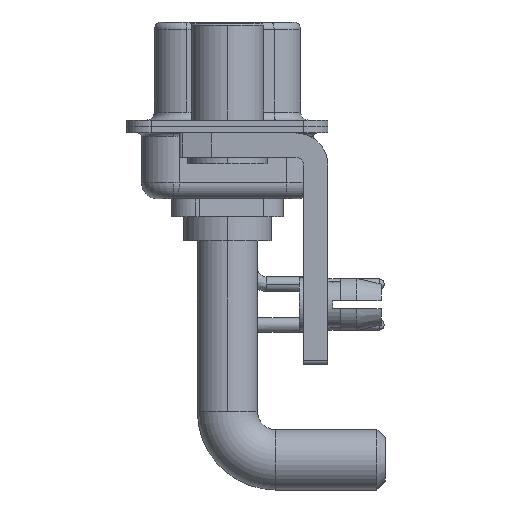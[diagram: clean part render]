
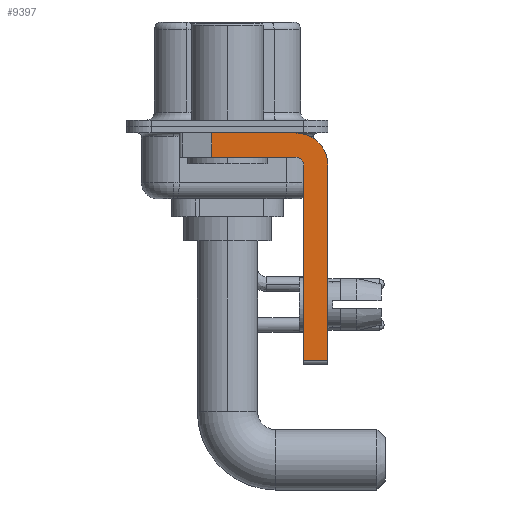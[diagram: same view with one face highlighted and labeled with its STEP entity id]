
A CAD part, left-side view. The second image highlights one B-rep face of the part: STEP entity #9397.
In plain terms, the highlighted planar face has unit normal (-1, 0, 0).
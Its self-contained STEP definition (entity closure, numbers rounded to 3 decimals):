
#890 = EDGE_CURVE ( 'NONE', #4836, #10333, #4775, .T. ) ;
#1061 = LINE ( 'NONE', #7834, #28828 ) ;
#1086 = VECTOR ( 'NONE', #16494, 1000. ) ;
#1589 = VECTOR ( 'NONE', #26887, 1000. ) ;
#1786 = CARTESIAN_POINT ( 'NONE',  ( -2.9, -6.25, -2.4 ) ) ;
#2987 = VECTOR ( 'NONE', #22084, 1000. ) ;
#4348 = CARTESIAN_POINT ( 'NONE',  ( -2.9, 0.978, -0.4 ) ) ;
#4496 = EDGE_CURVE ( 'NONE', #12629, #29725, #12776, .T. ) ;
#4773 = VERTEX_POINT ( 'NONE', #27335 ) ;
#4775 = LINE ( 'NONE', #1786, #22903 ) ;
#4836 = VERTEX_POINT ( 'NONE', #17969 ) ;
#4913 = CARTESIAN_POINT ( 'NONE',  ( -2.9, 3., -0.4 ) ) ;
#5280 = EDGE_CURVE ( 'NONE', #29725, #14616, #12431, .T. ) ;
#5698 = CARTESIAN_POINT ( 'NONE',  ( -2.9, -4.25, -2.4 ) ) ;
#6232 = CARTESIAN_POINT ( 'NONE',  ( -2.9, -4.25, -14.55 ) ) ;
#6456 = DIRECTION ( 'NONE',  ( -1., 0., 0. ) ) ;
#6915 = ORIENTED_EDGE ( 'NONE', *, *, #9900, .T. ) ;
#7355 = ORIENTED_EDGE ( 'NONE', *, *, #890, .F. ) ;
#7834 = CARTESIAN_POINT ( 'NONE',  ( -2.9, 0.978, -1.9 ) ) ;
#8520 = LINE ( 'NONE', #17688, #2987 ) ;
#8548 = PLANE ( 'NONE',  #23224 ) ;
#8713 = EDGE_CURVE ( 'NONE', #26566, #4836, #13050, .T. ) ;
#8742 = AXIS2_PLACEMENT_3D ( 'NONE', #5698, #9798, #18960 ) ;
#9298 = EDGE_LOOP ( 'NONE', ( #19048, #26282, #26952, #13839, #11290, #6915, #7355, #17602 ) ) ;
#9397 = ADVANCED_FACE ( 'NONE', ( #28735 ), #8548, .F. ) ;
#9798 = DIRECTION ( 'NONE',  ( 1., 0., 0. ) ) ;
#9900 = EDGE_CURVE ( 'NONE', #12629, #10333, #20096, .T. ) ;
#10202 = CARTESIAN_POINT ( 'NONE',  ( -2.9, -4.25, -0.4 ) ) ;
#10333 = VERTEX_POINT ( 'NONE', #24891 ) ;
#10504 = CARTESIAN_POINT ( 'NONE',  ( -2.9, -4.25, -2.4 ) ) ;
#10971 = AXIS2_PLACEMENT_3D ( 'NONE', #27119, #6456, #16095 ) ;
#11091 = EDGE_CURVE ( 'NONE', #14616, #4773, #8520, .T. ) ;
#11290 = ORIENTED_EDGE ( 'NONE', *, *, #4496, .F. ) ;
#12431 = CIRCLE ( 'NONE', #10971, 0.5 ) ;
#12629 = VERTEX_POINT ( 'NONE', #20824 ) ;
#12776 = LINE ( 'NONE', #19999, #20083 ) ;
#12793 = DIRECTION ( 'NONE',  ( 0., 0., -1. ) ) ;
#13050 = CIRCLE ( 'NONE', #8742, 2. ) ;
#13839 = ORIENTED_EDGE ( 'NONE', *, *, #5280, .F. ) ;
#14616 = VERTEX_POINT ( 'NONE', #23884 ) ;
#15623 = EDGE_CURVE ( 'NONE', #17021, #4773, #1061, .T. ) ;
#16095 = DIRECTION ( 'NONE',  ( 0., 0., 1. ) ) ;
#16494 = DIRECTION ( 'NONE',  ( 0., -1., 0. ) ) ;
#16785 = LINE ( 'NONE', #4913, #1086 ) ;
#17021 = VERTEX_POINT ( 'NONE', #4348 ) ;
#17573 = DIRECTION ( 'NONE',  ( 0., 0., -1. ) ) ;
#17602 = ORIENTED_EDGE ( 'NONE', *, *, #8713, .F. ) ;
#17688 = CARTESIAN_POINT ( 'NONE',  ( -2.9, -4.25, -1.9 ) ) ;
#17969 = CARTESIAN_POINT ( 'NONE',  ( -2.9, -6.25, -2.4 ) ) ;
#18960 = DIRECTION ( 'NONE',  ( 0., 0., -1. ) ) ;
#19048 = ORIENTED_EDGE ( 'NONE', *, *, #29455, .F. ) ;
#19999 = CARTESIAN_POINT ( 'NONE',  ( -2.9, -4.75, -14.8 ) ) ;
#20083 = VECTOR ( 'NONE', #24391, 1000. ) ;
#20096 = LINE ( 'NONE', #6232, #1589 ) ;
#20139 = DIRECTION ( 'NONE',  ( 0., 0., -1. ) ) ;
#20824 = CARTESIAN_POINT ( 'NONE',  ( -2.9, -4.75, -14.55 ) ) ;
#22084 = DIRECTION ( 'NONE',  ( 0., 1., 0. ) ) ;
#22903 = VECTOR ( 'NONE', #20139, 1000. ) ;
#23224 = AXIS2_PLACEMENT_3D ( 'NONE', #10504, #24378, #17573 ) ;
#23884 = CARTESIAN_POINT ( 'NONE',  ( -2.9, -4.25, -1.9 ) ) ;
#24378 = DIRECTION ( 'NONE',  ( 1., 0., 0. ) ) ;
#24391 = DIRECTION ( 'NONE',  ( 0., 0., 1. ) ) ;
#24891 = CARTESIAN_POINT ( 'NONE',  ( -2.9, -6.25, -14.55 ) ) ;
#25226 = CARTESIAN_POINT ( 'NONE',  ( -2.9, -4.75, -2.4 ) ) ;
#26282 = ORIENTED_EDGE ( 'NONE', *, *, #15623, .T. ) ;
#26566 = VERTEX_POINT ( 'NONE', #10202 ) ;
#26887 = DIRECTION ( 'NONE',  ( 0., -1., 0. ) ) ;
#26952 = ORIENTED_EDGE ( 'NONE', *, *, #11091, .F. ) ;
#27119 = CARTESIAN_POINT ( 'NONE',  ( -2.9, -4.25, -2.4 ) ) ;
#27335 = CARTESIAN_POINT ( 'NONE',  ( -2.9, 0.978, -1.9 ) ) ;
#28735 = FACE_OUTER_BOUND ( 'NONE', #9298, .T. ) ;
#28828 = VECTOR ( 'NONE', #12793, 1000. ) ;
#29455 = EDGE_CURVE ( 'NONE', #17021, #26566, #16785, .T. ) ;
#29725 = VERTEX_POINT ( 'NONE', #25226 ) ;
